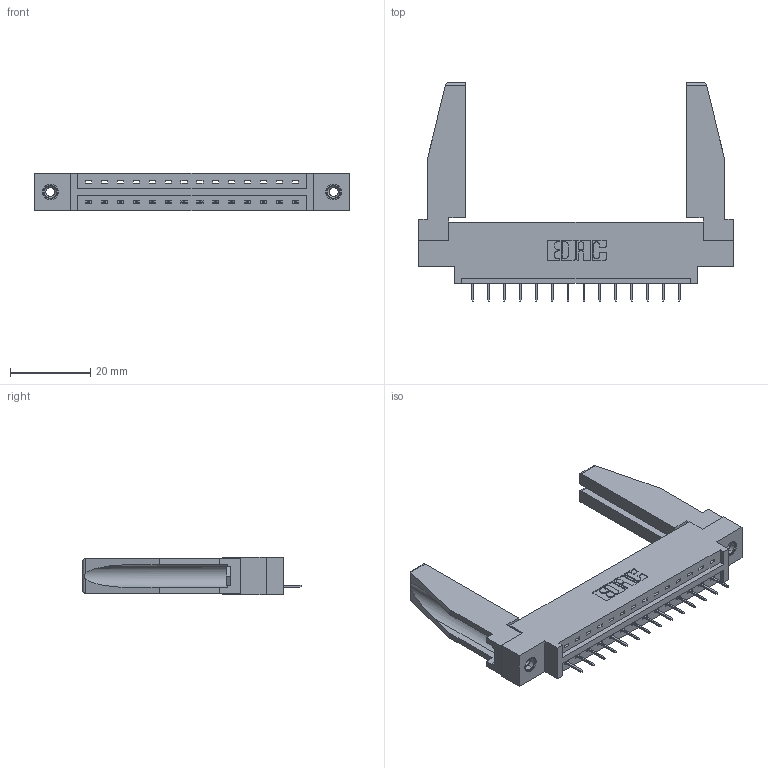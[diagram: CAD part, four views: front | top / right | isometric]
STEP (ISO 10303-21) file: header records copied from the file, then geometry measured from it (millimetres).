
FILE_DESCRIPTION (( 'STEP AP203' ), '1' );
FILE_NAME ('337-014-524-678.STEP', '2019-09-28T15:42:36', ( '' ), ( '' ), 'SwSTEP 2.0', 'SolidWorks 2016', '' );
FILE_SCHEMA (( 'CONFIG_CONTROL_DESIGN' ));
Length unit declared in the file: inch
Products named in the file (5): 337-014-524-678; 345-292-001_345-293-124; 307-220-078; 337 Part_0.170 Offset - 0.156 Dia-TI; 345-250-001_345-250-001-102
Assembly tree (19 placements, depth 2):
  337-014-524-678
    337 Part_0.170 Offset - 0.156 Dia-TI
    345-292-001_345-293-124  x14
    345-250-001_345-250-001-102  x2
    307-220-078  x2
Bounding box: 78.49 x 54.49 x 9.4 mm (x, y, z)
Volume: 11627.4 mm3; surface area: 11472.1 mm2
Topology: 19 solids, 19 shells, 1172 faces, 3341 edges, 2162 vertices
Faces by surface type: plane 886, cylinder 270, cone 12, torus 4
Entity records: 16674 total; most frequent: CARTESIAN_POINT 2894, ORIENTED_EDGE 2800, DIRECTION 2504, EDGE_CURVE 1400, LINE 1238, VECTOR 1238, VERTEX_POINT 924, AXIS2_PLACEMENT_3D 633
